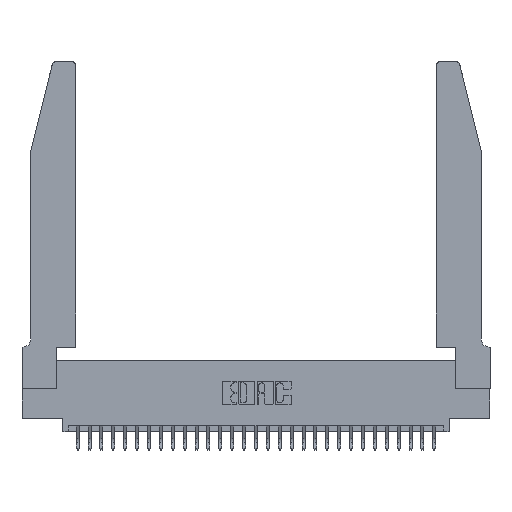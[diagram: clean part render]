
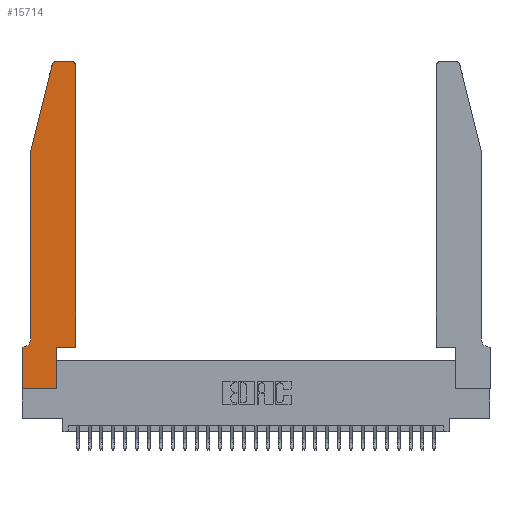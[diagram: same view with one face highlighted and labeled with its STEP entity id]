
A CAD part, top view. The second image highlights one B-rep face of the part: STEP entity #15714.
In plain terms, the highlighted planar face has unit normal (0, 0, 1).
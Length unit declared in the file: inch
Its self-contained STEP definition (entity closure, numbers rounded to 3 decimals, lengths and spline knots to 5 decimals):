
#84 = CARTESIAN_POINT ( 'NONE',  ( 0.2865, 0.35, 0.37 ) ) ;
#1185 = CARTESIAN_POINT ( 'NONE',  ( 0.0755, 2., 0.37 ) ) ;
#1188 = ORIENTED_EDGE ( 'NONE', *, *, #9500, .T. ) ;
#1210 = VERTEX_POINT ( 'NONE', #12472 ) ;
#1238 = CARTESIAN_POINT ( 'NONE',  ( 0.4505, 0.35, 0.37 ) ) ;
#1495 = ORIENTED_EDGE ( 'NONE', *, *, #15607, .T. ) ;
#1918 = CARTESIAN_POINT ( 'NONE',  ( 0.4505, 0.35, 0.37 ) ) ;
#1964 = EDGE_CURVE ( 'NONE', #7192, #1210, #14242, .T. ) ;
#2323 = CIRCLE ( 'NONE', #15536, 0.03 ) ;
#2869 = FACE_OUTER_BOUND ( 'NONE', #23444, .T. ) ;
#2929 = EDGE_CURVE ( 'NONE', #1210, #28728, #8578, .T. ) ;
#2950 = LINE ( 'NONE', #17791, #10178 ) ;
#3623 = LINE ( 'NONE', #16123, #21964 ) ;
#3658 = LINE ( 'NONE', #5125, #14201 ) ;
#4380 = DIRECTION ( 'NONE',  ( 1., 0., 0. ) ) ;
#4816 = LINE ( 'NONE', #1918, #20175 ) ;
#5125 = CARTESIAN_POINT ( 'NONE',  ( 0.2865, 0.35, 0.37 ) ) ;
#5164 = ORIENTED_EDGE ( 'NONE', *, *, #28569, .T. ) ;
#5824 = DIRECTION ( 'NONE',  ( 0., 1., 0. ) ) ;
#5905 = LINE ( 'NONE', #27916, #30422 ) ;
#6089 = CARTESIAN_POINT ( 'NONE',  ( 0., 0., 0.37 ) ) ;
#6563 = CIRCLE ( 'NONE', #15578, 0.03 ) ;
#6844 = DIRECTION ( 'NONE',  ( 0., -1., 0. ) ) ;
#6929 = ORIENTED_EDGE ( 'NONE', *, *, #26367, .T. ) ;
#6939 = LINE ( 'NONE', #1185, #29187 ) ;
#7142 = VECTOR ( 'NONE', #22654, 39.37008 ) ;
#7192 = VERTEX_POINT ( 'NONE', #22533 ) ;
#7366 = CARTESIAN_POINT ( 'NONE',  ( 0.4505, 2.72, 0.37 ) ) ;
#7576 = CARTESIAN_POINT ( 'NONE',  ( 0.0755, 0.35, 0.37 ) ) ;
#7842 = VECTOR ( 'NONE', #6844, 39.37008 ) ;
#8053 = CARTESIAN_POINT ( 'NONE',  ( 0.25487, 2.72718, 0.37 ) ) ;
#8578 = LINE ( 'NONE', #9261, #7842 ) ;
#8782 = EDGE_CURVE ( 'NONE', #13970, #29088, #2950, .T. ) ;
#9261 = CARTESIAN_POINT ( 'NONE',  ( 0., 0., 0.37 ) ) ;
#9500 = EDGE_CURVE ( 'NONE', #21993, #13970, #4816, .T. ) ;
#9718 = EDGE_CURVE ( 'NONE', #28666, #21993, #3658, .T. ) ;
#9832 = AXIS2_PLACEMENT_3D ( 'NONE', #24712, #10469, #27049 ) ;
#10142 = EDGE_CURVE ( 'NONE', #29929, #11690, #3623, .T. ) ;
#10178 = VECTOR ( 'NONE', #5824, 39.37008 ) ;
#10469 = DIRECTION ( 'NONE',  ( 0., 0., -1. ) ) ;
#10969 = DIRECTION ( 'NONE',  ( 0., -1., 0. ) ) ;
#11453 = CARTESIAN_POINT ( 'NONE',  ( 0.0755, 2., 0.37 ) ) ;
#11598 = CARTESIAN_POINT ( 'NONE',  ( 0.2605, 2.75, 0.37 ) ) ;
#11690 = VERTEX_POINT ( 'NONE', #11453 ) ;
#11701 = DIRECTION ( 'NONE',  ( 0., 0., 1. ) ) ;
#12472 = CARTESIAN_POINT ( 'NONE',  ( 0., 0.35, 0.37 ) ) ;
#13111 = ORIENTED_EDGE ( 'NONE', *, *, #10142, .T. ) ;
#13497 = CARTESIAN_POINT ( 'NONE',  ( 0.4205, 2.72, 0.37 ) ) ;
#13970 = VERTEX_POINT ( 'NONE', #1238 ) ;
#14010 = DIRECTION ( 'NONE',  ( -1., 0., 0. ) ) ;
#14076 = ORIENTED_EDGE ( 'NONE', *, *, #2929, .T. ) ;
#14201 = VECTOR ( 'NONE', #28923, 39.37008 ) ;
#14242 = LINE ( 'NONE', #7576, #7142 ) ;
#15536 = AXIS2_PLACEMENT_3D ( 'NONE', #13497, #30012, #15904 ) ;
#15578 = AXIS2_PLACEMENT_3D ( 'NONE', #25955, #11701, #28278 ) ;
#15607 = EDGE_CURVE ( 'NONE', #29539, #16330, #17206, .T. ) ;
#15714 = ADVANCED_FACE ( 'NONE', ( #2869 ), #19130, .T. ) ;
#15904 = DIRECTION ( 'NONE',  ( 1., 0., 0. ) ) ;
#15988 = AXIS2_PLACEMENT_3D ( 'NONE', #16739, #28464, #21478 ) ;
#16123 = CARTESIAN_POINT ( 'NONE',  ( 0.0755, 2., 0.37 ) ) ;
#16330 = VERTEX_POINT ( 'NONE', #16392 ) ;
#16392 = CARTESIAN_POINT ( 'NONE',  ( 0.284, 2.75, 0.37 ) ) ;
#16497 = ORIENTED_EDGE ( 'NONE', *, *, #9718, .T. ) ;
#16739 = CARTESIAN_POINT ( 'NONE',  ( 0., 0.35, 0.37 ) ) ;
#17206 = LINE ( 'NONE', #11598, #28972 ) ;
#17412 = ORIENTED_EDGE ( 'NONE', *, *, #21684, .T. ) ;
#17791 = CARTESIAN_POINT ( 'NONE',  ( 0.4505, 0.35, 0.37 ) ) ;
#19130 = PLANE ( 'NONE',  #15988 ) ;
#19706 = ORIENTED_EDGE ( 'NONE', *, *, #1964, .T. ) ;
#20175 = VECTOR ( 'NONE', #4380, 39.37008 ) ;
#20224 = ORIENTED_EDGE ( 'NONE', *, *, #24578, .T. ) ;
#20672 = VERTEX_POINT ( 'NONE', #28286 ) ;
#21072 = ORIENTED_EDGE ( 'NONE', *, *, #23941, .T. ) ;
#21478 = DIRECTION ( 'NONE',  ( 1., 0., 0. ) ) ;
#21684 = EDGE_CURVE ( 'NONE', #28728, #28666, #5905, .T. ) ;
#21964 = VECTOR ( 'NONE', #25658, 39.37008 ) ;
#21993 = VERTEX_POINT ( 'NONE', #84 ) ;
#22533 = CARTESIAN_POINT ( 'NONE',  ( 0.0055, 0.35, 0.37 ) ) ;
#22654 = DIRECTION ( 'NONE',  ( -1., 0., 0. ) ) ;
#23444 = EDGE_LOOP ( 'NONE', ( #1495, #6929, #13111, #20224, #5164, #19706, #14076, #17412, #16497, #1188, #24206, #21072 ) ) ;
#23941 = EDGE_CURVE ( 'NONE', #29088, #29539, #2323, .T. ) ;
#24206 = ORIENTED_EDGE ( 'NONE', *, *, #8782, .T. ) ;
#24578 = EDGE_CURVE ( 'NONE', #11690, #20672, #6939, .T. ) ;
#24712 = CARTESIAN_POINT ( 'NONE',  ( 0.0055, 0.42, 0.37 ) ) ;
#25593 = DIRECTION ( 'NONE',  ( 1., 0., 0. ) ) ;
#25658 = DIRECTION ( 'NONE',  ( -0.239, -0.971, 0. ) ) ;
#25955 = CARTESIAN_POINT ( 'NONE',  ( 0.284, 2.72, 0.37 ) ) ;
#26367 = EDGE_CURVE ( 'NONE', #16330, #29929, #6563, .T. ) ;
#27049 = DIRECTION ( 'NONE',  ( -1., 0., 0. ) ) ;
#27312 = CARTESIAN_POINT ( 'NONE',  ( 0.2865, 0., 0.37 ) ) ;
#27623 = CIRCLE ( 'NONE', #9832, 0.07 ) ;
#27762 = CARTESIAN_POINT ( 'NONE',  ( 0.4205, 2.75, 0.37 ) ) ;
#27916 = CARTESIAN_POINT ( 'NONE',  ( 0., 0., 0.37 ) ) ;
#28278 = DIRECTION ( 'NONE',  ( 1., 0., 0. ) ) ;
#28286 = CARTESIAN_POINT ( 'NONE',  ( 0.0755, 0.42, 0.37 ) ) ;
#28464 = DIRECTION ( 'NONE',  ( 0., 0., 1. ) ) ;
#28569 = EDGE_CURVE ( 'NONE', #20672, #7192, #27623, .T. ) ;
#28666 = VERTEX_POINT ( 'NONE', #27312 ) ;
#28728 = VERTEX_POINT ( 'NONE', #6089 ) ;
#28923 = DIRECTION ( 'NONE',  ( 0., 1., 0. ) ) ;
#28972 = VECTOR ( 'NONE', #14010, 39.37008 ) ;
#29088 = VERTEX_POINT ( 'NONE', #7366 ) ;
#29187 = VECTOR ( 'NONE', #10969, 39.37008 ) ;
#29539 = VERTEX_POINT ( 'NONE', #27762 ) ;
#29929 = VERTEX_POINT ( 'NONE', #8053 ) ;
#30012 = DIRECTION ( 'NONE',  ( 0., 0., 1. ) ) ;
#30422 = VECTOR ( 'NONE', #25593, 39.37008 ) ;
